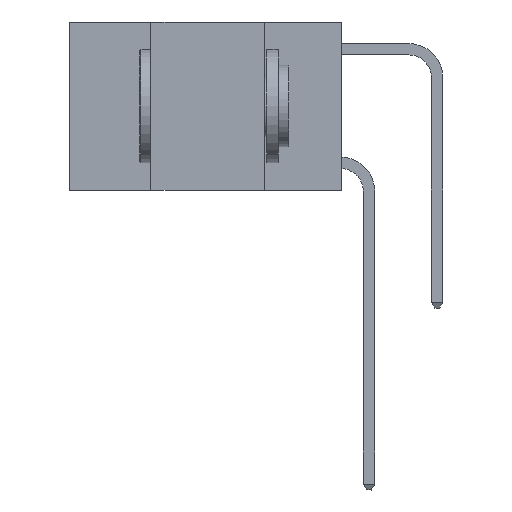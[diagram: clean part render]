
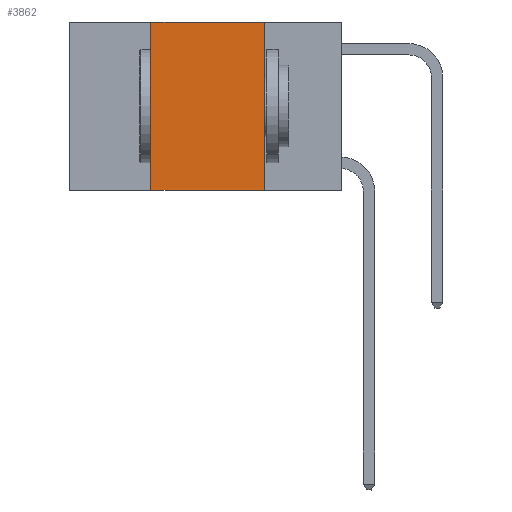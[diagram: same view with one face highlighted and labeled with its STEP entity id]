
A CAD part, left-side view. The second image highlights one B-rep face of the part: STEP entity #3862.
In plain terms, the highlighted planar face has unit normal (-1, 0, 0).
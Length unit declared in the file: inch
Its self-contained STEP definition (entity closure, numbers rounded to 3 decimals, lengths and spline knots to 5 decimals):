
#128 = CARTESIAN_POINT ( 'NONE',  ( 0., 0.42, 0. ) ) ;
#829 = CARTESIAN_POINT ( 'NONE',  ( 0., 0.42, 0. ) ) ;
#887 = CARTESIAN_POINT ( 'NONE',  ( 0., 0.6, -0.37 ) ) ;
#1106 = EDGE_CURVE ( 'NONE', #7125, #1547, #6946, .T. ) ;
#1547 = VERTEX_POINT ( 'NONE', #1853 ) ;
#1853 = CARTESIAN_POINT ( 'NONE',  ( 0., 0.17, 0. ) ) ;
#2030 = CARTESIAN_POINT ( 'NONE',  ( 0., 0.6, 0. ) ) ;
#2196 = LINE ( 'NONE', #128, #11418 ) ;
#2254 = DIRECTION ( 'NONE',  ( 0., 0., 1. ) ) ;
#3034 = VECTOR ( 'NONE', #8224, 39.37008 ) ;
#3678 = VERTEX_POINT ( 'NONE', #7299 ) ;
#3862 = ADVANCED_FACE ( 'NONE', ( #6476 ), #9551, .F. ) ;
#4084 = AXIS2_PLACEMENT_3D ( 'NONE', #8658, #5155, #11295 ) ;
#4340 = EDGE_CURVE ( 'NONE', #1547, #3678, #6183, .T. ) ;
#4586 = EDGE_LOOP ( 'NONE', ( #8907, #9849, #10474, #9607 ) ) ;
#4664 = DIRECTION ( 'NONE',  ( 0., -1., 0. ) ) ;
#5155 = DIRECTION ( 'NONE',  ( 1., 0., 0. ) ) ;
#5811 = CARTESIAN_POINT ( 'NONE',  ( 0., 0.42, -0.37 ) ) ;
#6183 = LINE ( 'NONE', #6656, #10860 ) ;
#6476 = FACE_OUTER_BOUND ( 'NONE', #4586, .T. ) ;
#6555 = VERTEX_POINT ( 'NONE', #5811 ) ;
#6615 = DIRECTION ( 'NONE',  ( 0., 0., -1. ) ) ;
#6656 = CARTESIAN_POINT ( 'NONE',  ( 0., 0.17, 0. ) ) ;
#6946 = LINE ( 'NONE', #2030, #9281 ) ;
#7125 = VERTEX_POINT ( 'NONE', #829 ) ;
#7299 = CARTESIAN_POINT ( 'NONE',  ( 0., 0.17, -0.37 ) ) ;
#8224 = DIRECTION ( 'NONE',  ( 0., -1., 0. ) ) ;
#8658 = CARTESIAN_POINT ( 'NONE',  ( 0., 0.6, 0. ) ) ;
#8907 = ORIENTED_EDGE ( 'NONE', *, *, #4340, .F. ) ;
#9281 = VECTOR ( 'NONE', #4664, 39.37008 ) ;
#9551 = PLANE ( 'NONE',  #4084 ) ;
#9607 = ORIENTED_EDGE ( 'NONE', *, *, #9719, .T. ) ;
#9719 = EDGE_CURVE ( 'NONE', #6555, #3678, #10355, .T. ) ;
#9849 = ORIENTED_EDGE ( 'NONE', *, *, #1106, .F. ) ;
#10355 = LINE ( 'NONE', #887, #3034 ) ;
#10474 = ORIENTED_EDGE ( 'NONE', *, *, #11647, .F. ) ;
#10860 = VECTOR ( 'NONE', #6615, 39.37008 ) ;
#11295 = DIRECTION ( 'NONE',  ( 0., 0., -1. ) ) ;
#11418 = VECTOR ( 'NONE', #2254, 39.37008 ) ;
#11647 = EDGE_CURVE ( 'NONE', #6555, #7125, #2196, .T. ) ;
